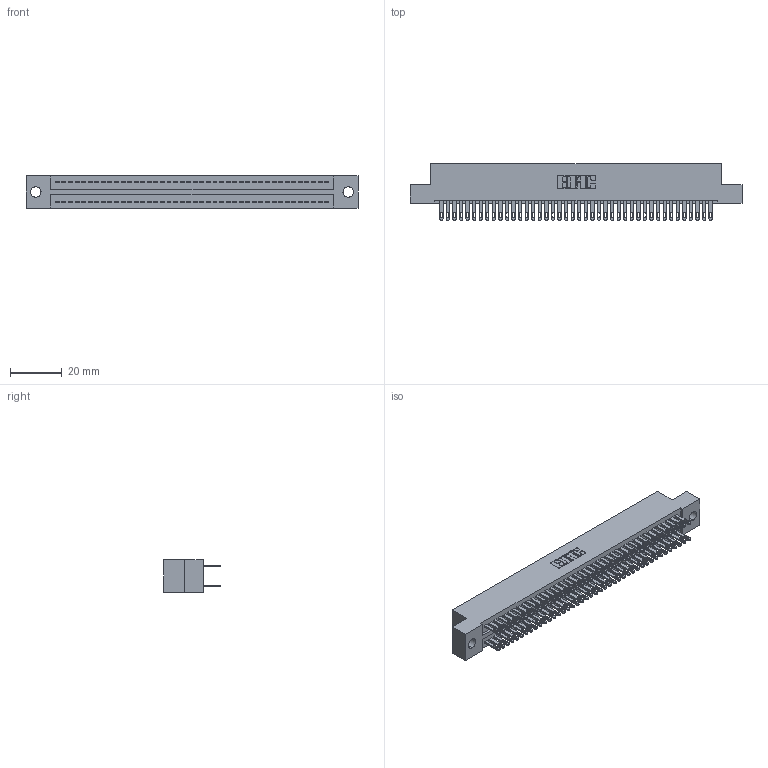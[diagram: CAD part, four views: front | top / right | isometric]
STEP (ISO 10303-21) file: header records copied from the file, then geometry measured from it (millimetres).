
FILE_DESCRIPTION (( 'STEP AP203' ), '1' );
FILE_NAME ('325-084-500-209.STEP', '2020-02-25T05:00:22', ( '' ), ( '' ), 'SwSTEP 2.0', 'SolidWorks 2016', '' );
FILE_SCHEMA (( 'CONFIG_CONTROL_DESIGN' ));
Length unit declared in the file: inch
Products named in the file (3): 325 Part_.160 TH; 325-084-500-209; 325-292-001_325-293-100
Assembly tree (85 placements, depth 2):
  325-084-500-209
    325 Part_.160 TH
    325-292-001_325-293-100  x84
Bounding box: 128.4 x 21.84 x 12.45 mm (x, y, z)
Volume: 16601.4 mm3; surface area: 20892.5 mm2
Topology: 85 solids, 85 shells, 4146 faces, 12659 edges, 8438 vertices
Faces by surface type: plane 2590, cylinder 1556
Entity records: 26953 total; most frequent: CARTESIAN_POINT 4466, ORIENTED_EDGE 4402, DIRECTION 3817, EDGE_CURVE 2201, LINE 2069, VECTOR 2069, VERTEX_POINT 1466, AXIS2_PLACEMENT_3D 874
